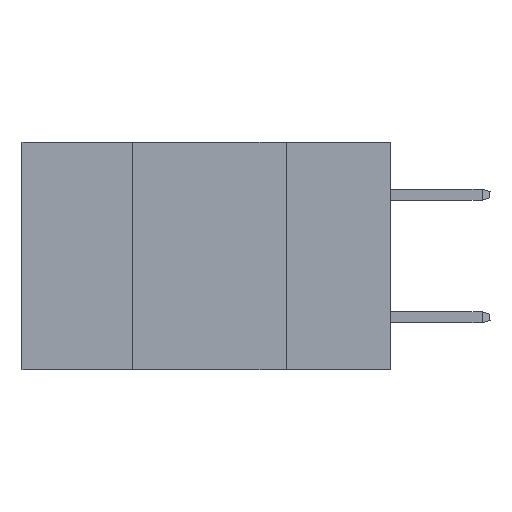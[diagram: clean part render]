
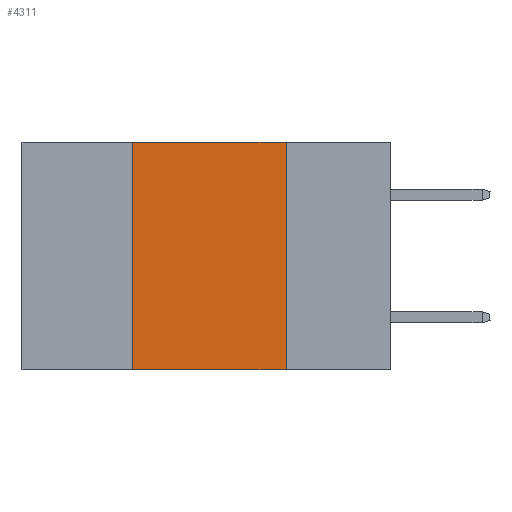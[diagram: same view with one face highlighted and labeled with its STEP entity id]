
A CAD part, left-side view. The second image highlights one B-rep face of the part: STEP entity #4311.
In plain terms, the highlighted planar face has unit normal (-1, 0, 0).
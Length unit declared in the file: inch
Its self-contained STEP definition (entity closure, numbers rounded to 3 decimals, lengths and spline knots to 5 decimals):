
#226 = VECTOR ( 'NONE', #4027, 39.37008 ) ;
#660 = DIRECTION ( 'NONE',  ( 0., 0., -1. ) ) ;
#942 = EDGE_CURVE ( 'NONE', #6552, #12040, #4515, .T. ) ;
#1134 = ORIENTED_EDGE ( 'NONE', *, *, #11592, .F. ) ;
#1144 = DIRECTION ( 'NONE',  ( 0., 0., 1. ) ) ;
#1485 = AXIS2_PLACEMENT_3D ( 'NONE', #4988, #4851, #660 ) ;
#1848 = CARTESIAN_POINT ( 'NONE',  ( 0., 0.42, -0.37 ) ) ;
#2648 = ORIENTED_EDGE ( 'NONE', *, *, #942, .T. ) ;
#2972 = CARTESIAN_POINT ( 'NONE',  ( 0., 0.6, -0.37 ) ) ;
#3399 = CARTESIAN_POINT ( 'NONE',  ( 0., 0.17, -0.37 ) ) ;
#3832 = VERTEX_POINT ( 'NONE', #5177 ) ;
#3911 = ORIENTED_EDGE ( 'NONE', *, *, #8575, .F. ) ;
#4027 = DIRECTION ( 'NONE',  ( 0., -1., 0. ) ) ;
#4311 = ADVANCED_FACE ( 'NONE', ( #8865 ), #11144, .F. ) ;
#4515 = LINE ( 'NONE', #2972, #226 ) ;
#4851 = DIRECTION ( 'NONE',  ( 1., 0., 0. ) ) ;
#4988 = CARTESIAN_POINT ( 'NONE',  ( 0., 0.6, 0. ) ) ;
#5088 = CARTESIAN_POINT ( 'NONE',  ( 0., 0.42, 0. ) ) ;
#5177 = CARTESIAN_POINT ( 'NONE',  ( 0., 0.17, 0. ) ) ;
#6290 = CARTESIAN_POINT ( 'NONE',  ( 0., 0.6, 0. ) ) ;
#6516 = ORIENTED_EDGE ( 'NONE', *, *, #8537, .F. ) ;
#6552 = VERTEX_POINT ( 'NONE', #1848 ) ;
#6840 = VERTEX_POINT ( 'NONE', #5088 ) ;
#7357 = DIRECTION ( 'NONE',  ( 0., -1., 0. ) ) ;
#7756 = CARTESIAN_POINT ( 'NONE',  ( 0., 0.17, 0. ) ) ;
#8055 = EDGE_LOOP ( 'NONE', ( #1134, #6516, #3911, #2648 ) ) ;
#8537 = EDGE_CURVE ( 'NONE', #6840, #3832, #11051, .T. ) ;
#8575 = EDGE_CURVE ( 'NONE', #6552, #6840, #8721, .T. ) ;
#8721 = LINE ( 'NONE', #11608, #11685 ) ;
#8865 = FACE_OUTER_BOUND ( 'NONE', #8055, .T. ) ;
#11051 = LINE ( 'NONE', #6290, #12807 ) ;
#11144 = PLANE ( 'NONE',  #1485 ) ;
#11592 = EDGE_CURVE ( 'NONE', #3832, #12040, #12968, .T. ) ;
#11608 = CARTESIAN_POINT ( 'NONE',  ( 0., 0.42, 0. ) ) ;
#11685 = VECTOR ( 'NONE', #1144, 39.37008 ) ;
#11988 = VECTOR ( 'NONE', #12962, 39.37008 ) ;
#12040 = VERTEX_POINT ( 'NONE', #3399 ) ;
#12807 = VECTOR ( 'NONE', #7357, 39.37008 ) ;
#12962 = DIRECTION ( 'NONE',  ( 0., 0., -1. ) ) ;
#12968 = LINE ( 'NONE', #7756, #11988 ) ;
